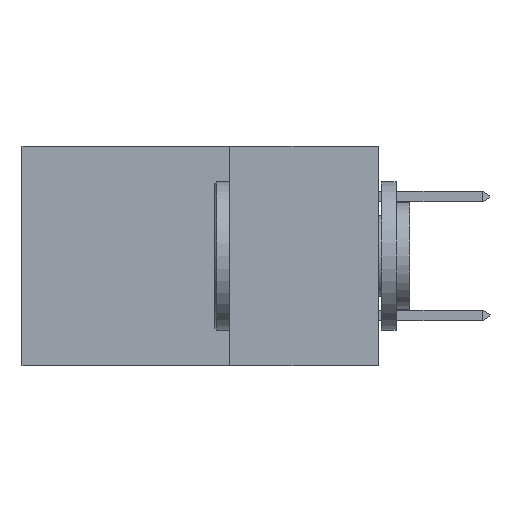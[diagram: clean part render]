
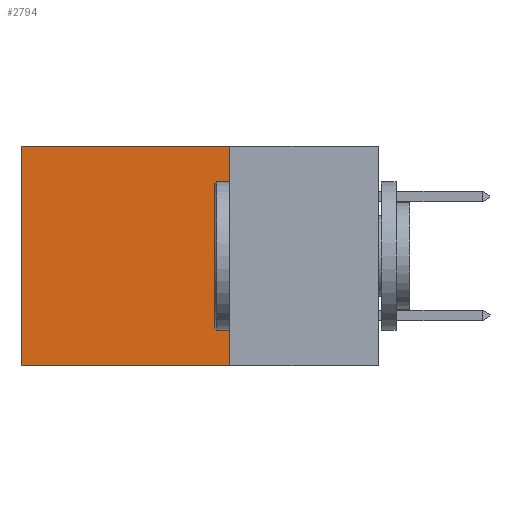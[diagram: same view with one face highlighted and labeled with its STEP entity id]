
A CAD part, left-side view. The second image highlights one B-rep face of the part: STEP entity #2794.
In plain terms, the highlighted planar face has unit normal (-1, 0, 0).
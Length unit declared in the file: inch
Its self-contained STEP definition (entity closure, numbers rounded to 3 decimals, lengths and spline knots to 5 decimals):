
#682 = CARTESIAN_POINT ( 'NONE',  ( 0.298, 0.6, 0. ) ) ;
#1078 = CARTESIAN_POINT ( 'NONE',  ( 0.298, 0.25, 0. ) ) ;
#2634 = DIRECTION ( 'NONE',  ( 0., 1., 0. ) ) ;
#2740 = FACE_OUTER_BOUND ( 'NONE', #16057, .T. ) ;
#2741 = DIRECTION ( 'NONE',  ( 0., 0., -1. ) ) ;
#2794 = ADVANCED_FACE ( 'NONE', ( #2740 ), #14596, .F. ) ;
#3107 = LINE ( 'NONE', #17560, #9525 ) ;
#4515 = DIRECTION ( 'NONE',  ( 0., 1., 0. ) ) ;
#5038 = VERTEX_POINT ( 'NONE', #682 ) ;
#5720 = CARTESIAN_POINT ( 'NONE',  ( 0.298, 0.25, 0. ) ) ;
#5969 = VECTOR ( 'NONE', #2634, 39.37008 ) ;
#6562 = EDGE_CURVE ( 'NONE', #5038, #9921, #3107, .T. ) ;
#8641 = CARTESIAN_POINT ( 'NONE',  ( 0.298, 0.25, 0. ) ) ;
#9525 = VECTOR ( 'NONE', #11709, 39.37008 ) ;
#9724 = VECTOR ( 'NONE', #18746, 39.37008 ) ;
#9921 = VERTEX_POINT ( 'NONE', #11406 ) ;
#10565 = LINE ( 'NONE', #18304, #18207 ) ;
#10727 = EDGE_CURVE ( 'NONE', #10780, #5038, #18111, .T. ) ;
#10780 = VERTEX_POINT ( 'NONE', #1078 ) ;
#11203 = EDGE_CURVE ( 'NONE', #10780, #17191, #16425, .T. ) ;
#11231 = ORIENTED_EDGE ( 'NONE', *, *, #10727, .T. ) ;
#11406 = CARTESIAN_POINT ( 'NONE',  ( 0.298, 0.6, -0.37 ) ) ;
#11482 = DIRECTION ( 'NONE',  ( 1., 0., 0. ) ) ;
#11709 = DIRECTION ( 'NONE',  ( 0., 0., -1. ) ) ;
#14596 = PLANE ( 'NONE',  #17887 ) ;
#14887 = ORIENTED_EDGE ( 'NONE', *, *, #6562, .T. ) ;
#15314 = ORIENTED_EDGE ( 'NONE', *, *, #19733, .F. ) ;
#15627 = CARTESIAN_POINT ( 'NONE',  ( 0.298, 0.25, -0.37 ) ) ;
#16057 = EDGE_LOOP ( 'NONE', ( #14887, #15314, #16703, #11231 ) ) ;
#16425 = LINE ( 'NONE', #18603, #9724 ) ;
#16703 = ORIENTED_EDGE ( 'NONE', *, *, #11203, .F. ) ;
#17191 = VERTEX_POINT ( 'NONE', #15627 ) ;
#17560 = CARTESIAN_POINT ( 'NONE',  ( 0.298, 0.6, 0. ) ) ;
#17887 = AXIS2_PLACEMENT_3D ( 'NONE', #8641, #11482, #2741 ) ;
#18111 = LINE ( 'NONE', #5720, #5969 ) ;
#18207 = VECTOR ( 'NONE', #4515, 39.37008 ) ;
#18304 = CARTESIAN_POINT ( 'NONE',  ( 0.298, 0.25, -0.37 ) ) ;
#18603 = CARTESIAN_POINT ( 'NONE',  ( 0.298, 0.25, 0. ) ) ;
#18746 = DIRECTION ( 'NONE',  ( 0., 0., -1. ) ) ;
#19733 = EDGE_CURVE ( 'NONE', #17191, #9921, #10565, .T. ) ;
